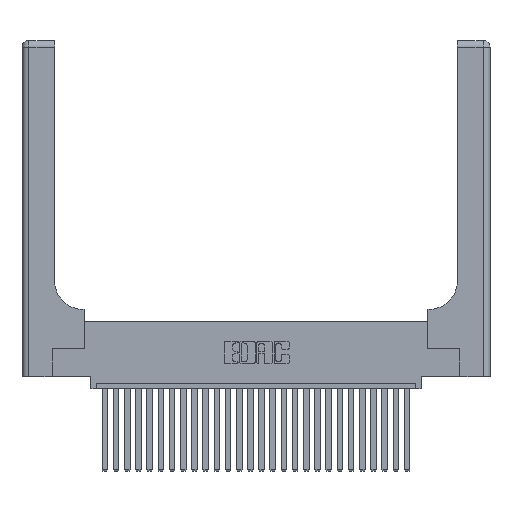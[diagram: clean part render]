
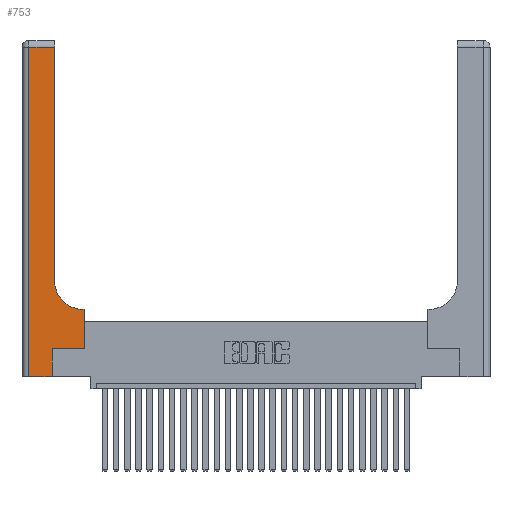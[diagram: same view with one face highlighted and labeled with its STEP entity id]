
A CAD part, top view. The second image highlights one B-rep face of the part: STEP entity #753.
In plain terms, the highlighted planar face has unit normal (0, 0, 1).
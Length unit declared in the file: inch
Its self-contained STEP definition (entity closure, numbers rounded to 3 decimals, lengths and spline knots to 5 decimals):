
#100 = AXIS2_PLACEMENT_3D ( 'NONE', #25819, #17058, #1806 ) ;
#143 = DIRECTION ( 'NONE',  ( -1., 0., 0. ) ) ;
#266 = CARTESIAN_POINT ( 'NONE',  ( 0., 0., 0.37 ) ) ;
#278 = DIRECTION ( 'NONE',  ( 0., -1., 0. ) ) ;
#753 = ADVANCED_FACE ( 'NONE', ( #2117 ), #21626, .F. ) ;
#1688 = LINE ( 'NONE', #27916, #19059 ) ;
#1730 = CARTESIAN_POINT ( 'NONE',  ( 0.2915, 2.94, 0.37 ) ) ;
#1752 = VECTOR ( 'NONE', #17076, 39.37008 ) ;
#1806 = DIRECTION ( 'NONE',  ( 1., 0., 0. ) ) ;
#1820 = CARTESIAN_POINT ( 'NONE',  ( 0., 2.94, 0.37 ) ) ;
#2007 = VECTOR ( 'NONE', #7654, 39.37008 ) ;
#2117 = FACE_OUTER_BOUND ( 'NONE', #7557, .T. ) ;
#2265 = VERTEX_POINT ( 'NONE', #12362 ) ;
#2341 = EDGE_CURVE ( 'NONE', #6249, #21140, #1688, .T. ) ;
#2971 = CARTESIAN_POINT ( 'NONE',  ( 0.269, 0.25, 0.37 ) ) ;
#3077 = CARTESIAN_POINT ( 'NONE',  ( 0.269, 0., 0.37 ) ) ;
#3746 = EDGE_CURVE ( 'NONE', #4204, #10227, #8516, .T. ) ;
#4204 = VERTEX_POINT ( 'NONE', #3077 ) ;
#4237 = VERTEX_POINT ( 'NONE', #5888 ) ;
#4443 = DIRECTION ( 'NONE',  ( 1., 0., 0. ) ) ;
#4785 = CARTESIAN_POINT ( 'NONE',  ( 0.06, 3., 0.37 ) ) ;
#5178 = VECTOR ( 'NONE', #278, 39.37008 ) ;
#5482 = CARTESIAN_POINT ( 'NONE',  ( 0.2915, 0.6, 0.37 ) ) ;
#5702 = VECTOR ( 'NONE', #4443, 39.37008 ) ;
#5888 = CARTESIAN_POINT ( 'NONE',  ( 0.06, 0., 0.37 ) ) ;
#6249 = VERTEX_POINT ( 'NONE', #9524 ) ;
#7557 = EDGE_LOOP ( 'NONE', ( #8333, #9011, #10366, #20706, #21405, #8239, #27937, #24419, #14328 ) ) ;
#7654 = DIRECTION ( 'NONE',  ( -1., 0., 0. ) ) ;
#7958 = EDGE_CURVE ( 'NONE', #14121, #17141, #10669, .T. ) ;
#8239 = ORIENTED_EDGE ( 'NONE', *, *, #12051, .T. ) ;
#8333 = ORIENTED_EDGE ( 'NONE', *, *, #20920, .T. ) ;
#8516 = LINE ( 'NONE', #10660, #16651 ) ;
#8737 = CARTESIAN_POINT ( 'NONE',  ( 0.269, 0.25, 0.37 ) ) ;
#8843 = DIRECTION ( 'NONE',  ( 0., 0., -1. ) ) ;
#9011 = ORIENTED_EDGE ( 'NONE', *, *, #24537, .T. ) ;
#9155 = DIRECTION ( 'NONE',  ( 1., 0., 0. ) ) ;
#9455 = EDGE_CURVE ( 'NONE', #21140, #14121, #16348, .T. ) ;
#9524 = CARTESIAN_POINT ( 'NONE',  ( 0.5585, 0.25, 0.37 ) ) ;
#10227 = VERTEX_POINT ( 'NONE', #2971 ) ;
#10366 = ORIENTED_EDGE ( 'NONE', *, *, #24857, .T. ) ;
#10660 = CARTESIAN_POINT ( 'NONE',  ( 0.269, 0., 0.37 ) ) ;
#10669 = CIRCLE ( 'NONE', #100, 0.25 ) ;
#11357 = CARTESIAN_POINT ( 'NONE',  ( 0.2915, 3., 0.37 ) ) ;
#12051 = EDGE_CURVE ( 'NONE', #10227, #6249, #19626, .T. ) ;
#12362 = CARTESIAN_POINT ( 'NONE',  ( 0.06, 2.94, 0.37 ) ) ;
#13072 = VERTEX_POINT ( 'NONE', #1730 ) ;
#14121 = VERTEX_POINT ( 'NONE', #27919 ) ;
#14328 = ORIENTED_EDGE ( 'NONE', *, *, #7958, .T. ) ;
#14565 = LINE ( 'NONE', #266, #19949 ) ;
#16272 = LINE ( 'NONE', #11357, #24695 ) ;
#16348 = LINE ( 'NONE', #5482, #2007 ) ;
#16651 = VECTOR ( 'NONE', #21534, 39.37008 ) ;
#17058 = DIRECTION ( 'NONE',  ( 0., 0., -1. ) ) ;
#17076 = DIRECTION ( 'NONE',  ( -1., 0., 0. ) ) ;
#17141 = VERTEX_POINT ( 'NONE', #20439 ) ;
#17464 = AXIS2_PLACEMENT_3D ( 'NONE', #23791, #8843, #143 ) ;
#17957 = DIRECTION ( 'NONE',  ( 0., 1., 0. ) ) ;
#19059 = VECTOR ( 'NONE', #21357, 39.37008 ) ;
#19108 = LINE ( 'NONE', #4785, #5178 ) ;
#19626 = LINE ( 'NONE', #8737, #5702 ) ;
#19949 = VECTOR ( 'NONE', #9155, 39.37008 ) ;
#20439 = CARTESIAN_POINT ( 'NONE',  ( 0.2915, 0.85, 0.37 ) ) ;
#20706 = ORIENTED_EDGE ( 'NONE', *, *, #22064, .T. ) ;
#20920 = EDGE_CURVE ( 'NONE', #17141, #13072, #16272, .T. ) ;
#21140 = VERTEX_POINT ( 'NONE', #22541 ) ;
#21357 = DIRECTION ( 'NONE',  ( 0., 1., 0. ) ) ;
#21405 = ORIENTED_EDGE ( 'NONE', *, *, #3746, .T. ) ;
#21534 = DIRECTION ( 'NONE',  ( 0., 1., 0. ) ) ;
#21626 = PLANE ( 'NONE',  #17464 ) ;
#22064 = EDGE_CURVE ( 'NONE', #4237, #4204, #14565, .T. ) ;
#22541 = CARTESIAN_POINT ( 'NONE',  ( 0.5585, 0.6, 0.37 ) ) ;
#23791 = CARTESIAN_POINT ( 'NONE',  ( 0., 3., 0.37 ) ) ;
#24419 = ORIENTED_EDGE ( 'NONE', *, *, #9455, .T. ) ;
#24537 = EDGE_CURVE ( 'NONE', #13072, #2265, #24836, .T. ) ;
#24695 = VECTOR ( 'NONE', #17957, 39.37008 ) ;
#24836 = LINE ( 'NONE', #1820, #1752 ) ;
#24857 = EDGE_CURVE ( 'NONE', #2265, #4237, #19108, .T. ) ;
#25819 = CARTESIAN_POINT ( 'NONE',  ( 0.5415, 0.85, 0.37 ) ) ;
#27916 = CARTESIAN_POINT ( 'NONE',  ( 0.5585, 0.25, 0.37 ) ) ;
#27919 = CARTESIAN_POINT ( 'NONE',  ( 0.5415, 0.6, 0.37 ) ) ;
#27937 = ORIENTED_EDGE ( 'NONE', *, *, #2341, .T. ) ;
